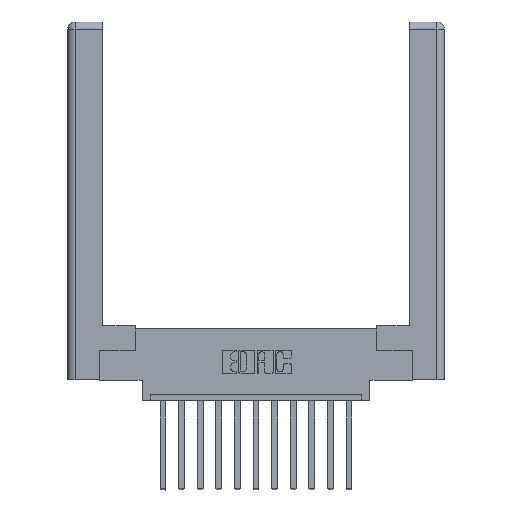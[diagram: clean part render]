
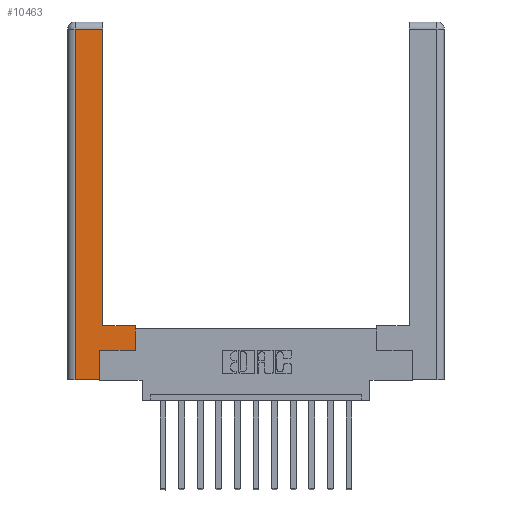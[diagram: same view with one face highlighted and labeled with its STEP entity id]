
A CAD part, top view. The second image highlights one B-rep face of the part: STEP entity #10463.
In plain terms, the highlighted planar face has unit normal (0, 0, 1).
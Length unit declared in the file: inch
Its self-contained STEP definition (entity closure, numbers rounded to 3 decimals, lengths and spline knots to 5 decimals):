
#438 = LINE ( 'NONE', #1414, #3463 ) ;
#904 = LINE ( 'NONE', #7180, #6602 ) ;
#1030 = ORIENTED_EDGE ( 'NONE', *, *, #5688, .T. ) ;
#1131 = DIRECTION ( 'NONE',  ( 0., -1., 0. ) ) ;
#1294 = CARTESIAN_POINT ( 'NONE',  ( 0.565, 0.245, 0. ) ) ;
#1334 = VERTEX_POINT ( 'NONE', #13735 ) ;
#1414 = CARTESIAN_POINT ( 'NONE',  ( 0.265, 0., 0. ) ) ;
#1439 = VERTEX_POINT ( 'NONE', #14041 ) ;
#1954 = EDGE_CURVE ( 'NONE', #8409, #14015, #8309, .T. ) ;
#1981 = ORIENTED_EDGE ( 'NONE', *, *, #3312, .T. ) ;
#2171 = EDGE_CURVE ( 'NONE', #10396, #1439, #10673, .T. ) ;
#2578 = VERTEX_POINT ( 'NONE', #1294 ) ;
#2910 = VECTOR ( 'NONE', #10612, 39.37008 ) ;
#3296 = CARTESIAN_POINT ( 'NONE',  ( 0.0615, 0., 0. ) ) ;
#3312 = EDGE_CURVE ( 'NONE', #4479, #9808, #3531, .T. ) ;
#3463 = VECTOR ( 'NONE', #12535, 39.37008 ) ;
#3531 = LINE ( 'NONE', #3296, #14595 ) ;
#3812 = CARTESIAN_POINT ( 'NONE',  ( 0.265, 0.245, 0. ) ) ;
#3898 = CARTESIAN_POINT ( 'NONE',  ( 0.0615, 0., 0. ) ) ;
#4479 = VERTEX_POINT ( 'NONE', #8132 ) ;
#4646 = DIRECTION ( 'NONE',  ( -1., 0., 0. ) ) ;
#4686 = DIRECTION ( 'NONE',  ( 0., 0., -1. ) ) ;
#4726 = CARTESIAN_POINT ( 'NONE',  ( 0.295, 0.45, 0. ) ) ;
#5489 = EDGE_CURVE ( 'NONE', #14015, #1334, #6849, .T. ) ;
#5563 = CARTESIAN_POINT ( 'NONE',  ( 0.295, 3., 0. ) ) ;
#5688 = EDGE_CURVE ( 'NONE', #9808, #10396, #438, .T. ) ;
#5694 = CARTESIAN_POINT ( 'NONE',  ( 0.0615, 2.94, 0. ) ) ;
#5883 = ORIENTED_EDGE ( 'NONE', *, *, #7355, .T. ) ;
#6602 = VECTOR ( 'NONE', #13205, 39.37008 ) ;
#6747 = VECTOR ( 'NONE', #11714, 39.37008 ) ;
#6825 = DIRECTION ( 'NONE',  ( -1., 0., 0. ) ) ;
#6849 = LINE ( 'NONE', #5563, #12170 ) ;
#7121 = CARTESIAN_POINT ( 'NONE',  ( 0., 0., 0. ) ) ;
#7180 = CARTESIAN_POINT ( 'NONE',  ( 0.565, 0.45, 0. ) ) ;
#7355 = EDGE_CURVE ( 'NONE', #1439, #2578, #12821, .T. ) ;
#7411 = ORIENTED_EDGE ( 'NONE', *, *, #5489, .T. ) ;
#8052 = EDGE_CURVE ( 'NONE', #1334, #4479, #14097, .T. ) ;
#8132 = CARTESIAN_POINT ( 'NONE',  ( 0.0615, 2.94, 0. ) ) ;
#8162 = PLANE ( 'NONE',  #13070 ) ;
#8309 = LINE ( 'NONE', #9309, #12938 ) ;
#8409 = VERTEX_POINT ( 'NONE', #13952 ) ;
#9309 = CARTESIAN_POINT ( 'NONE',  ( 0.295, 0.45, 0. ) ) ;
#9808 = VERTEX_POINT ( 'NONE', #3898 ) ;
#9922 = ORIENTED_EDGE ( 'NONE', *, *, #2171, .T. ) ;
#10396 = VERTEX_POINT ( 'NONE', #13711 ) ;
#10463 = ADVANCED_FACE ( 'NONE', ( #11268 ), #8162, .F. ) ;
#10612 = DIRECTION ( 'NONE',  ( 1., 0., 0. ) ) ;
#10673 = LINE ( 'NONE', #3812, #6747 ) ;
#11036 = VECTOR ( 'NONE', #6825, 39.37008 ) ;
#11268 = FACE_OUTER_BOUND ( 'NONE', #14545, .T. ) ;
#11714 = DIRECTION ( 'NONE',  ( 0., 1., 0. ) ) ;
#11784 = ORIENTED_EDGE ( 'NONE', *, *, #8052, .T. ) ;
#12170 = VECTOR ( 'NONE', #14468, 39.37008 ) ;
#12535 = DIRECTION ( 'NONE',  ( 1., 0., 0. ) ) ;
#12620 = DIRECTION ( 'NONE',  ( -1., 0., 0. ) ) ;
#12682 = EDGE_CURVE ( 'NONE', #2578, #8409, #904, .T. ) ;
#12821 = LINE ( 'NONE', #12840, #2910 ) ;
#12840 = CARTESIAN_POINT ( 'NONE',  ( 0.565, 0.245, 0. ) ) ;
#12938 = VECTOR ( 'NONE', #4646, 39.37008 ) ;
#13070 = AXIS2_PLACEMENT_3D ( 'NONE', #7121, #4686, #12620 ) ;
#13183 = ORIENTED_EDGE ( 'NONE', *, *, #1954, .T. ) ;
#13205 = DIRECTION ( 'NONE',  ( 0., 1., 0. ) ) ;
#13711 = CARTESIAN_POINT ( 'NONE',  ( 0.265, 0., 0. ) ) ;
#13735 = CARTESIAN_POINT ( 'NONE',  ( 0.295, 2.94, 0. ) ) ;
#13753 = ORIENTED_EDGE ( 'NONE', *, *, #12682, .T. ) ;
#13952 = CARTESIAN_POINT ( 'NONE',  ( 0.565, 0.45, 0. ) ) ;
#14015 = VERTEX_POINT ( 'NONE', #4726 ) ;
#14041 = CARTESIAN_POINT ( 'NONE',  ( 0.265, 0.245, 0. ) ) ;
#14097 = LINE ( 'NONE', #5694, #11036 ) ;
#14468 = DIRECTION ( 'NONE',  ( 0., 1., 0. ) ) ;
#14545 = EDGE_LOOP ( 'NONE', ( #7411, #11784, #1981, #1030, #9922, #5883, #13753, #13183 ) ) ;
#14595 = VECTOR ( 'NONE', #1131, 39.37008 ) ;
